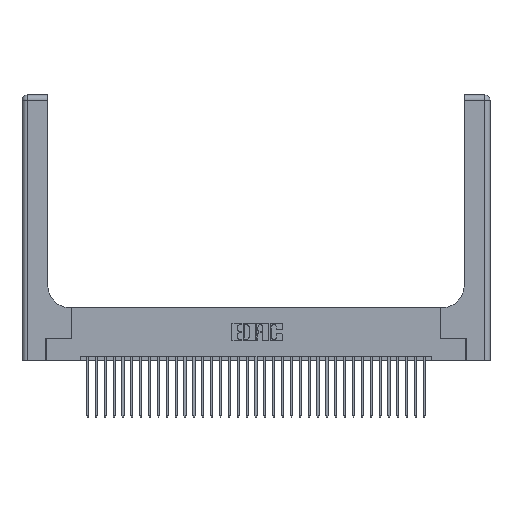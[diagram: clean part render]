
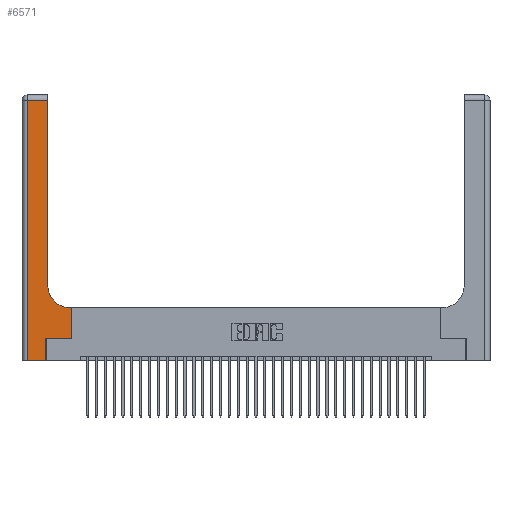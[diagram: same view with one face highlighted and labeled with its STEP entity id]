
A CAD part, top view. The second image highlights one B-rep face of the part: STEP entity #6571.
In plain terms, the highlighted planar face has unit normal (0, 0, 1).
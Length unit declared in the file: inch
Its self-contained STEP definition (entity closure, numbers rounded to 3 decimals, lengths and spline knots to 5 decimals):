
#147 = VERTEX_POINT ( 'NONE', #34470 ) ;
#447 = VECTOR ( 'NONE', #1468, 39.37008 ) ;
#530 = DIRECTION ( 'NONE',  ( 0., -1., 0. ) ) ;
#1192 = DIRECTION ( 'NONE',  ( 0., 1., 0. ) ) ;
#1468 = DIRECTION ( 'NONE',  ( -1., 0., 0. ) ) ;
#1663 = LINE ( 'NONE', #19541, #15698 ) ;
#1698 = VECTOR ( 'NONE', #1192, 39.37008 ) ;
#1896 = VERTEX_POINT ( 'NONE', #19488 ) ;
#2521 = ORIENTED_EDGE ( 'NONE', *, *, #4373, .T. ) ;
#2727 = DIRECTION ( 'NONE',  ( 1., 0., 0. ) ) ;
#3280 = ORIENTED_EDGE ( 'NONE', *, *, #24854, .T. ) ;
#3699 = VECTOR ( 'NONE', #530, 39.37008 ) ;
#4373 = EDGE_CURVE ( 'NONE', #13508, #27699, #26057, .T. ) ;
#4525 = CARTESIAN_POINT ( 'NONE',  ( 0.5585, 0.25, 0.37 ) ) ;
#4856 = EDGE_CURVE ( 'NONE', #20335, #28569, #25638, .T. ) ;
#4879 = CARTESIAN_POINT ( 'NONE',  ( 0.5585, 0.25, 0.37 ) ) ;
#6225 = CARTESIAN_POINT ( 'NONE',  ( 0.5415, 0.6, 0.37 ) ) ;
#6571 = ADVANCED_FACE ( 'NONE', ( #14099 ), #12657, .F. ) ;
#7116 = CARTESIAN_POINT ( 'NONE',  ( 0.2915, 0.85, 0.37 ) ) ;
#7268 = EDGE_CURVE ( 'NONE', #18265, #13508, #22831, .T. ) ;
#7895 = EDGE_CURVE ( 'NONE', #25383, #18265, #9167, .T. ) ;
#8361 = EDGE_CURVE ( 'NONE', #1896, #147, #1663, .T. ) ;
#8982 = CARTESIAN_POINT ( 'NONE',  ( 0.06, 3., 0.37 ) ) ;
#9167 = LINE ( 'NONE', #31888, #1698 ) ;
#9726 = CARTESIAN_POINT ( 'NONE',  ( 0., 3., 0.37 ) ) ;
#10208 = AXIS2_PLACEMENT_3D ( 'NONE', #36200, #19501, #2727 ) ;
#10747 = EDGE_CURVE ( 'NONE', #28569, #25383, #12897, .T. ) ;
#11237 = ORIENTED_EDGE ( 'NONE', *, *, #7895, .T. ) ;
#11547 = AXIS2_PLACEMENT_3D ( 'NONE', #9726, #15482, #35000 ) ;
#11753 = ORIENTED_EDGE ( 'NONE', *, *, #34992, .T. ) ;
#11785 = CARTESIAN_POINT ( 'NONE',  ( 0.5585, 0.6, 0.37 ) ) ;
#12657 = PLANE ( 'NONE',  #11547 ) ;
#12897 = CIRCLE ( 'NONE', #10208, 0.25 ) ;
#12916 = EDGE_CURVE ( 'NONE', #27699, #1896, #32164, .T. ) ;
#13508 = VERTEX_POINT ( 'NONE', #33162 ) ;
#14099 = FACE_OUTER_BOUND ( 'NONE', #34906, .T. ) ;
#15440 = CARTESIAN_POINT ( 'NONE',  ( 0., 2.94, 0.37 ) ) ;
#15482 = DIRECTION ( 'NONE',  ( 0., 0., -1. ) ) ;
#15698 = VECTOR ( 'NONE', #22354, 39.37008 ) ;
#16093 = CARTESIAN_POINT ( 'NONE',  ( 0.269, 0.25, 0.37 ) ) ;
#16388 = ORIENTED_EDGE ( 'NONE', *, *, #7268, .T. ) ;
#16533 = DIRECTION ( 'NONE',  ( -1., 0., 0. ) ) ;
#18265 = VERTEX_POINT ( 'NONE', #24917 ) ;
#19036 = VECTOR ( 'NONE', #16533, 39.37008 ) ;
#19124 = CARTESIAN_POINT ( 'NONE',  ( 0.06, 0., 0.37 ) ) ;
#19421 = CARTESIAN_POINT ( 'NONE',  ( 0., 0., 0.37 ) ) ;
#19488 = CARTESIAN_POINT ( 'NONE',  ( 0.269, 0., 0.37 ) ) ;
#19501 = DIRECTION ( 'NONE',  ( 0., 0., -1. ) ) ;
#19541 = CARTESIAN_POINT ( 'NONE',  ( 0.269, 0., 0.37 ) ) ;
#20335 = VERTEX_POINT ( 'NONE', #11785 ) ;
#20408 = VECTOR ( 'NONE', #21283, 39.37008 ) ;
#21283 = DIRECTION ( 'NONE',  ( 0., 1., 0. ) ) ;
#22354 = DIRECTION ( 'NONE',  ( 0., 1., 0. ) ) ;
#22831 = LINE ( 'NONE', #15440, #447 ) ;
#23226 = VECTOR ( 'NONE', #30031, 39.37008 ) ;
#23897 = VECTOR ( 'NONE', #25075, 39.37008 ) ;
#24854 = EDGE_CURVE ( 'NONE', #147, #26417, #24981, .T. ) ;
#24917 = CARTESIAN_POINT ( 'NONE',  ( 0.2915, 2.94, 0.37 ) ) ;
#24981 = LINE ( 'NONE', #16093, #23226 ) ;
#25075 = DIRECTION ( 'NONE',  ( 1., 0., 0. ) ) ;
#25383 = VERTEX_POINT ( 'NONE', #7116 ) ;
#25638 = LINE ( 'NONE', #33266, #19036 ) ;
#26057 = LINE ( 'NONE', #8982, #3699 ) ;
#26417 = VERTEX_POINT ( 'NONE', #4879 ) ;
#26740 = ORIENTED_EDGE ( 'NONE', *, *, #8361, .T. ) ;
#27557 = ORIENTED_EDGE ( 'NONE', *, *, #10747, .T. ) ;
#27658 = ORIENTED_EDGE ( 'NONE', *, *, #12916, .T. ) ;
#27699 = VERTEX_POINT ( 'NONE', #19124 ) ;
#28569 = VERTEX_POINT ( 'NONE', #6225 ) ;
#30031 = DIRECTION ( 'NONE',  ( 1., 0., 0. ) ) ;
#30891 = ORIENTED_EDGE ( 'NONE', *, *, #4856, .T. ) ;
#31888 = CARTESIAN_POINT ( 'NONE',  ( 0.2915, 3., 0.37 ) ) ;
#32164 = LINE ( 'NONE', #19421, #23897 ) ;
#33162 = CARTESIAN_POINT ( 'NONE',  ( 0.06, 2.94, 0.37 ) ) ;
#33266 = CARTESIAN_POINT ( 'NONE',  ( 0.2915, 0.6, 0.37 ) ) ;
#34358 = LINE ( 'NONE', #4525, #20408 ) ;
#34470 = CARTESIAN_POINT ( 'NONE',  ( 0.269, 0.25, 0.37 ) ) ;
#34906 = EDGE_LOOP ( 'NONE', ( #11237, #16388, #2521, #27658, #26740, #3280, #11753, #30891, #27557 ) ) ;
#34992 = EDGE_CURVE ( 'NONE', #26417, #20335, #34358, .T. ) ;
#35000 = DIRECTION ( 'NONE',  ( -1., 0., 0. ) ) ;
#36200 = CARTESIAN_POINT ( 'NONE',  ( 0.5415, 0.85, 0.37 ) ) ;
